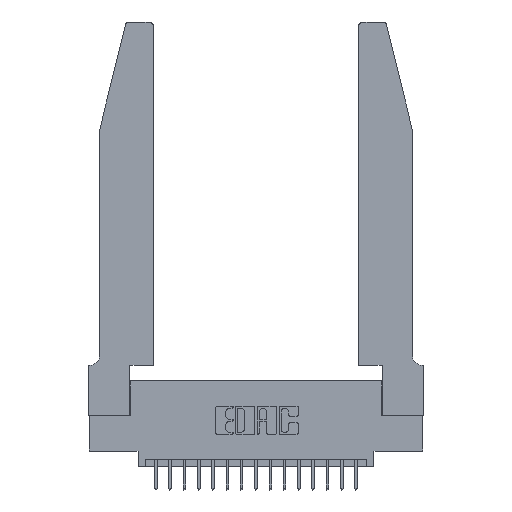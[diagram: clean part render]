
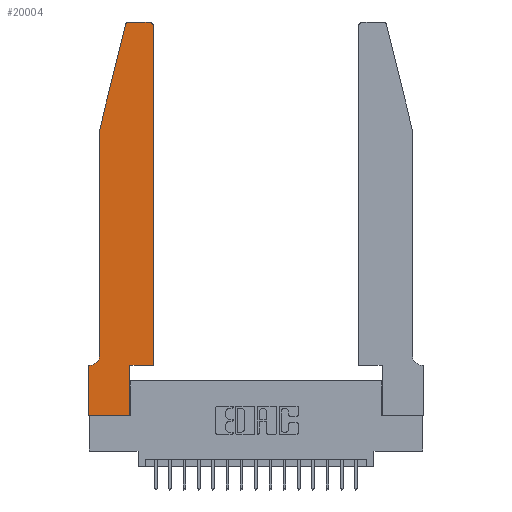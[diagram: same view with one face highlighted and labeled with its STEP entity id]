
A CAD part, top view. The second image highlights one B-rep face of the part: STEP entity #20004.
In plain terms, the highlighted planar face has unit normal (0, 0, 1).
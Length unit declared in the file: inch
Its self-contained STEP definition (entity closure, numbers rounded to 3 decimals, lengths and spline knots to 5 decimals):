
#96 = CARTESIAN_POINT ( 'NONE',  ( 0.4205, 2.72, 0.37 ) ) ;
#308 = LINE ( 'NONE', #1581, #4007 ) ;
#317 = VERTEX_POINT ( 'NONE', #15960 ) ;
#470 = LINE ( 'NONE', #14394, #12676 ) ;
#526 = CARTESIAN_POINT ( 'NONE',  ( 0., 0.35, 0.37 ) ) ;
#542 = EDGE_CURVE ( 'NONE', #4782, #14858, #5408, .T. ) ;
#851 = EDGE_CURVE ( 'NONE', #18923, #317, #3608, .T. ) ;
#856 = ORIENTED_EDGE ( 'NONE', *, *, #16638, .T. ) ;
#900 = EDGE_CURVE ( 'NONE', #12251, #18923, #6383, .T. ) ;
#1149 = VECTOR ( 'NONE', #10284, 39.37008 ) ;
#1479 = DIRECTION ( 'NONE',  ( 1., 0., 0. ) ) ;
#1581 = CARTESIAN_POINT ( 'NONE',  ( 0.0755, 0.35, 0.37 ) ) ;
#1668 = DIRECTION ( 'NONE',  ( 1., 0., 0. ) ) ;
#1737 = DIRECTION ( 'NONE',  ( 1., 0., 0. ) ) ;
#2101 = VECTOR ( 'NONE', #4378, 39.37008 ) ;
#2236 = VERTEX_POINT ( 'NONE', #12402 ) ;
#2314 = ORIENTED_EDGE ( 'NONE', *, *, #851, .T. ) ;
#2683 = EDGE_CURVE ( 'NONE', #9747, #5286, #19354, .T. ) ;
#3079 = CARTESIAN_POINT ( 'NONE',  ( 0.25487, 2.72718, 0.37 ) ) ;
#3580 = CARTESIAN_POINT ( 'NONE',  ( 0.0055, 0.35, 0.37 ) ) ;
#3608 = LINE ( 'NONE', #5004, #7400 ) ;
#3729 = AXIS2_PLACEMENT_3D ( 'NONE', #13807, #4273, #15374 ) ;
#4007 = VECTOR ( 'NONE', #11157, 39.37008 ) ;
#4058 = VERTEX_POINT ( 'NONE', #13141 ) ;
#4273 = DIRECTION ( 'NONE',  ( 0., 0., 1. ) ) ;
#4378 = DIRECTION ( 'NONE',  ( -0.239, -0.971, 0. ) ) ;
#4420 = CARTESIAN_POINT ( 'NONE',  ( 0.0755, 2., 0.37 ) ) ;
#4782 = VERTEX_POINT ( 'NONE', #526 ) ;
#4949 = CARTESIAN_POINT ( 'NONE',  ( 0.4505, 0.35, 0.37 ) ) ;
#4985 = CARTESIAN_POINT ( 'NONE',  ( 0.4205, 2.75, 0.37 ) ) ;
#5004 = CARTESIAN_POINT ( 'NONE',  ( 0.0755, 2., 0.37 ) ) ;
#5076 = DIRECTION ( 'NONE',  ( 0., -1., 0. ) ) ;
#5192 = VECTOR ( 'NONE', #7155, 39.37008 ) ;
#5286 = VERTEX_POINT ( 'NONE', #4949 ) ;
#5408 = LINE ( 'NONE', #8313, #1149 ) ;
#6010 = ORIENTED_EDGE ( 'NONE', *, *, #2683, .T. ) ;
#6383 = LINE ( 'NONE', #4420, #2101 ) ;
#6486 = ORIENTED_EDGE ( 'NONE', *, *, #9028, .T. ) ;
#6534 = DIRECTION ( 'NONE',  ( 0., 0., -1. ) ) ;
#7082 = DIRECTION ( 'NONE',  ( 0., 1., 0. ) ) ;
#7155 = DIRECTION ( 'NONE',  ( -1., 0., 0. ) ) ;
#7300 = DIRECTION ( 'NONE',  ( 0., 0., 1. ) ) ;
#7400 = VECTOR ( 'NONE', #5076, 39.37008 ) ;
#7627 = CARTESIAN_POINT ( 'NONE',  ( 0., 0., 0.37 ) ) ;
#7764 = ORIENTED_EDGE ( 'NONE', *, *, #12058, .T. ) ;
#8125 = CIRCLE ( 'NONE', #3729, 0.03 ) ;
#8313 = CARTESIAN_POINT ( 'NONE',  ( 0., 0., 0.37 ) ) ;
#8371 = VECTOR ( 'NONE', #1479, 39.37008 ) ;
#8540 = CIRCLE ( 'NONE', #15323, 0.03 ) ;
#8616 = ORIENTED_EDGE ( 'NONE', *, *, #19707, .T. ) ;
#9028 = EDGE_CURVE ( 'NONE', #5286, #2236, #16990, .T. ) ;
#9723 = CARTESIAN_POINT ( 'NONE',  ( 0.4505, 0.35, 0.37 ) ) ;
#9747 = VERTEX_POINT ( 'NONE', #10930 ) ;
#9856 = EDGE_CURVE ( 'NONE', #18135, #9747, #470, .T. ) ;
#10284 = DIRECTION ( 'NONE',  ( 0., -1., 0. ) ) ;
#10930 = CARTESIAN_POINT ( 'NONE',  ( 0.2865, 0.35, 0.37 ) ) ;
#11157 = DIRECTION ( 'NONE',  ( -1., 0., 0. ) ) ;
#11241 = DIRECTION ( 'NONE',  ( 0., 0., 1. ) ) ;
#11778 = VERTEX_POINT ( 'NONE', #3580 ) ;
#11811 = CARTESIAN_POINT ( 'NONE',  ( 0.4505, 0.35, 0.37 ) ) ;
#12058 = EDGE_CURVE ( 'NONE', #4058, #12251, #8125, .T. ) ;
#12242 = EDGE_CURVE ( 'NONE', #14858, #18135, #17193, .T. ) ;
#12251 = VERTEX_POINT ( 'NONE', #3079 ) ;
#12402 = CARTESIAN_POINT ( 'NONE',  ( 0.4505, 2.72, 0.37 ) ) ;
#12647 = CARTESIAN_POINT ( 'NONE',  ( 0., 0., 0.37 ) ) ;
#12676 = VECTOR ( 'NONE', #15927, 39.37008 ) ;
#13141 = CARTESIAN_POINT ( 'NONE',  ( 0.284, 2.75, 0.37 ) ) ;
#13416 = ORIENTED_EDGE ( 'NONE', *, *, #542, .T. ) ;
#13807 = CARTESIAN_POINT ( 'NONE',  ( 0.284, 2.72, 0.37 ) ) ;
#13896 = CIRCLE ( 'NONE', #17055, 0.07 ) ;
#14394 = CARTESIAN_POINT ( 'NONE',  ( 0.2865, 0.35, 0.37 ) ) ;
#14432 = EDGE_CURVE ( 'NONE', #2236, #19748, #8540, .T. ) ;
#14858 = VERTEX_POINT ( 'NONE', #7627 ) ;
#15098 = CARTESIAN_POINT ( 'NONE',  ( 0., 0.35, 0.37 ) ) ;
#15143 = ORIENTED_EDGE ( 'NONE', *, *, #14432, .T. ) ;
#15323 = AXIS2_PLACEMENT_3D ( 'NONE', #96, #11241, #1668 ) ;
#15374 = DIRECTION ( 'NONE',  ( 1., 0., 0. ) ) ;
#15816 = FACE_OUTER_BOUND ( 'NONE', #19910, .T. ) ;
#15927 = DIRECTION ( 'NONE',  ( 0., 1., 0. ) ) ;
#15960 = CARTESIAN_POINT ( 'NONE',  ( 0.0755, 0.42, 0.37 ) ) ;
#15967 = CARTESIAN_POINT ( 'NONE',  ( 0.0055, 0.42, 0.37 ) ) ;
#16500 = VECTOR ( 'NONE', #7082, 39.37008 ) ;
#16574 = CARTESIAN_POINT ( 'NONE',  ( 0.2605, 2.75, 0.37 ) ) ;
#16638 = EDGE_CURVE ( 'NONE', #11778, #4782, #308, .T. ) ;
#16710 = PLANE ( 'NONE',  #18718 ) ;
#16990 = LINE ( 'NONE', #11811, #16500 ) ;
#17050 = ORIENTED_EDGE ( 'NONE', *, *, #12242, .T. ) ;
#17055 = AXIS2_PLACEMENT_3D ( 'NONE', #15967, #6534, #17521 ) ;
#17193 = LINE ( 'NONE', #12647, #8371 ) ;
#17272 = LINE ( 'NONE', #16574, #5192 ) ;
#17521 = DIRECTION ( 'NONE',  ( -1., 0., 0. ) ) ;
#17859 = ORIENTED_EDGE ( 'NONE', *, *, #900, .T. ) ;
#17945 = ORIENTED_EDGE ( 'NONE', *, *, #9856, .T. ) ;
#18135 = VERTEX_POINT ( 'NONE', #19430 ) ;
#18256 = DIRECTION ( 'NONE',  ( 1., 0., 0. ) ) ;
#18718 = AXIS2_PLACEMENT_3D ( 'NONE', #15098, #7300, #18256 ) ;
#18923 = VERTEX_POINT ( 'NONE', #19794 ) ;
#19354 = LINE ( 'NONE', #9723, #19826 ) ;
#19430 = CARTESIAN_POINT ( 'NONE',  ( 0.2865, 0., 0.37 ) ) ;
#19707 = EDGE_CURVE ( 'NONE', #317, #11778, #13896, .T. ) ;
#19748 = VERTEX_POINT ( 'NONE', #4985 ) ;
#19794 = CARTESIAN_POINT ( 'NONE',  ( 0.0755, 2., 0.37 ) ) ;
#19826 = VECTOR ( 'NONE', #1737, 39.37008 ) ;
#19910 = EDGE_LOOP ( 'NONE', ( #19969, #7764, #17859, #2314, #8616, #856, #13416, #17050, #17945, #6010, #6486, #15143 ) ) ;
#19932 = EDGE_CURVE ( 'NONE', #19748, #4058, #17272, .T. ) ;
#19969 = ORIENTED_EDGE ( 'NONE', *, *, #19932, .T. ) ;
#20004 = ADVANCED_FACE ( 'NONE', ( #15816 ), #16710, .T. ) ;
